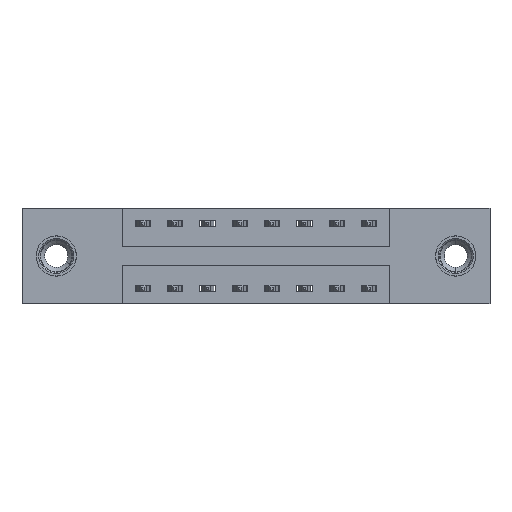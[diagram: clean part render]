
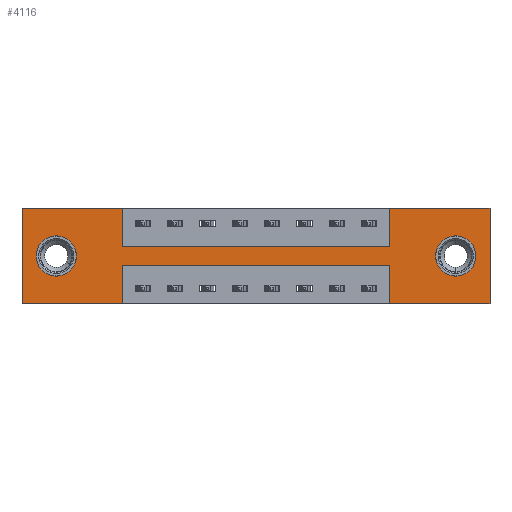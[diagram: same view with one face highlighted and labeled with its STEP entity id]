
A CAD part, front view. The second image highlights one B-rep face of the part: STEP entity #4116.
In plain terms, the highlighted planar face has unit normal (0, -1, 0).
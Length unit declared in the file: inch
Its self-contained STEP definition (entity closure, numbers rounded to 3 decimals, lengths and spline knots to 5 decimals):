
#4 = ORIENTED_EDGE ( 'NONE', *, *, #4979, .F. ) ;
#27 = CARTESIAN_POINT ( 'NONE',  ( 0., 0., -0.37 ) ) ;
#252 = LINE ( 'NONE', #2544, #3985 ) ;
#310 = LINE ( 'NONE', #9482, #10179 ) ;
#577 = ORIENTED_EDGE ( 'NONE', *, *, #8491, .F. ) ;
#803 = VECTOR ( 'NONE', #3928, 39.37008 ) ;
#817 = DIRECTION ( 'NONE',  ( 0., 0., 1. ) ) ;
#970 = AXIS2_PLACEMENT_3D ( 'NONE', #9080, #3993, #2358 ) ;
#1025 = CARTESIAN_POINT ( 'NONE',  ( 1.4225, 0., -0.37 ) ) ;
#1041 = ORIENTED_EDGE ( 'NONE', *, *, #8080, .F. ) ;
#1174 = CARTESIAN_POINT ( 'NONE',  ( 1.81, 0., 0. ) ) ;
#1250 = EDGE_CURVE ( 'NONE', #7081, #10296, #3600, .T. ) ;
#1262 = CARTESIAN_POINT ( 'NONE',  ( 0., 0., 0. ) ) ;
#1289 = ORIENTED_EDGE ( 'NONE', *, *, #5564, .F. ) ;
#1310 = CARTESIAN_POINT ( 'NONE',  ( 1.4225, 0., 0. ) ) ;
#1351 = CARTESIAN_POINT ( 'NONE',  ( 0.1325, 0., -0.185 ) ) ;
#1687 = CIRCLE ( 'NONE', #8643, 0.078 ) ;
#1735 = LINE ( 'NONE', #1174, #8257 ) ;
#1762 = ORIENTED_EDGE ( 'NONE', *, *, #9929, .F. ) ;
#1812 = DIRECTION ( 'NONE',  ( -1., 0., 0. ) ) ;
#1877 = VERTEX_POINT ( 'NONE', #9160 ) ;
#2152 = DIRECTION ( 'NONE',  ( 0., 1., 0. ) ) ;
#2358 = DIRECTION ( 'NONE',  ( 0., 0., 1. ) ) ;
#2379 = ORIENTED_EDGE ( 'NONE', *, *, #8146, .F. ) ;
#2544 = CARTESIAN_POINT ( 'NONE',  ( 0., 0., 0. ) ) ;
#2576 = CARTESIAN_POINT ( 'NONE',  ( 1.6775, 0., -0.185 ) ) ;
#2598 = EDGE_CURVE ( 'NONE', #11024, #10884, #2639, .T. ) ;
#2613 = CIRCLE ( 'NONE', #4164, 0.078 ) ;
#2615 = CARTESIAN_POINT ( 'NONE',  ( 1.4225, 0., 0. ) ) ;
#2639 = CIRCLE ( 'NONE', #5781, 0.078 ) ;
#2711 = VECTOR ( 'NONE', #8893, 39.37008 ) ;
#2727 = CARTESIAN_POINT ( 'NONE',  ( 0.1325, 0., -0.107 ) ) ;
#2881 = VECTOR ( 'NONE', #817, 39.37008 ) ;
#2910 = ORIENTED_EDGE ( 'NONE', *, *, #4052, .F. ) ;
#2995 = DIRECTION ( 'NONE',  ( 0., 0., 1. ) ) ;
#3021 = DIRECTION ( 'NONE',  ( 0., 1., 0. ) ) ;
#3043 = VERTEX_POINT ( 'NONE', #1025 ) ;
#3366 = DIRECTION ( 'NONE',  ( 0., -1., 0. ) ) ;
#3600 = LINE ( 'NONE', #3935, #6920 ) ;
#3783 = AXIS2_PLACEMENT_3D ( 'NONE', #27, #3366, #5979 ) ;
#3785 = EDGE_CURVE ( 'NONE', #10884, #11024, #2613, .T. ) ;
#3799 = DIRECTION ( 'NONE',  ( 1., 0., 0. ) ) ;
#3928 = DIRECTION ( 'NONE',  ( -1., 0., 0. ) ) ;
#3935 = CARTESIAN_POINT ( 'NONE',  ( 0.3875, 0., -0.37 ) ) ;
#3985 = VECTOR ( 'NONE', #8494, 39.37008 ) ;
#3993 = DIRECTION ( 'NONE',  ( 0., 1., 0. ) ) ;
#4052 = EDGE_CURVE ( 'NONE', #3043, #4626, #8217, .T. ) ;
#4082 = CARTESIAN_POINT ( 'NONE',  ( 0.3875, 0., -0.15 ) ) ;
#4116 = ADVANCED_FACE ( 'NONE', ( #9292, #9939, #6868 ), #10155, .T. ) ;
#4138 = CARTESIAN_POINT ( 'NONE',  ( 1.4225, 0., -0.37 ) ) ;
#4164 = AXIS2_PLACEMENT_3D ( 'NONE', #8963, #2152, #7339 ) ;
#4240 = VERTEX_POINT ( 'NONE', #6987 ) ;
#4421 = CARTESIAN_POINT ( 'NONE',  ( 0.3875, 0., -0.15 ) ) ;
#4422 = CARTESIAN_POINT ( 'NONE',  ( 0., 0., 0. ) ) ;
#4454 = LINE ( 'NONE', #1310, #5899 ) ;
#4476 = EDGE_CURVE ( 'NONE', #6394, #10966, #1687, .T. ) ;
#4532 = DIRECTION ( 'NONE',  ( 0., 0., -1. ) ) ;
#4626 = VERTEX_POINT ( 'NONE', #7547 ) ;
#4632 = CARTESIAN_POINT ( 'NONE',  ( 0.1325, 0., -0.263 ) ) ;
#4727 = ORIENTED_EDGE ( 'NONE', *, *, #3785, .T. ) ;
#4742 = VERTEX_POINT ( 'NONE', #8520 ) ;
#4807 = DIRECTION ( 'NONE',  ( 0., 0., -1. ) ) ;
#4900 = EDGE_CURVE ( 'NONE', #4742, #6120, #9551, .T. ) ;
#4979 = EDGE_CURVE ( 'NONE', #7237, #4742, #5648, .T. ) ;
#5195 = LINE ( 'NONE', #8920, #803 ) ;
#5290 = DIRECTION ( 'NONE',  ( 1., 0., 0. ) ) ;
#5388 = CARTESIAN_POINT ( 'NONE',  ( 0., 0., -0.37 ) ) ;
#5518 = ORIENTED_EDGE ( 'NONE', *, *, #2598, .T. ) ;
#5527 = VECTOR ( 'NONE', #4532, 39.37008 ) ;
#5564 = EDGE_CURVE ( 'NONE', #6120, #9863, #8842, .T. ) ;
#5648 = LINE ( 'NONE', #1262, #7539 ) ;
#5781 = AXIS2_PLACEMENT_3D ( 'NONE', #2576, #10335, #6895 ) ;
#5830 = CARTESIAN_POINT ( 'NONE',  ( 0.3875, 0., -0.37 ) ) ;
#5850 = CARTESIAN_POINT ( 'NONE',  ( 0.3875, 0., -0.22 ) ) ;
#5899 = VECTOR ( 'NONE', #10069, 39.37008 ) ;
#5979 = DIRECTION ( 'NONE',  ( 0., 0., -1. ) ) ;
#6120 = VERTEX_POINT ( 'NONE', #4421 ) ;
#6195 = CIRCLE ( 'NONE', #970, 0.078 ) ;
#6284 = EDGE_LOOP ( 'NONE', ( #5518, #4727 ) ) ;
#6394 = VERTEX_POINT ( 'NONE', #4632 ) ;
#6531 = ORIENTED_EDGE ( 'NONE', *, *, #4476, .T. ) ;
#6647 = ORIENTED_EDGE ( 'NONE', *, *, #10310, .F. ) ;
#6750 = EDGE_LOOP ( 'NONE', ( #6873, #2379, #2910, #577, #1041, #1762, #6647, #1289, #9093, #4, #9134, #6837 ) ) ;
#6837 = ORIENTED_EDGE ( 'NONE', *, *, #9474, .F. ) ;
#6861 = ORIENTED_EDGE ( 'NONE', *, *, #9233, .T. ) ;
#6868 = FACE_OUTER_BOUND ( 'NONE', #6750, .T. ) ;
#6873 = ORIENTED_EDGE ( 'NONE', *, *, #1250, .F. ) ;
#6895 = DIRECTION ( 'NONE',  ( 0., 0., -1. ) ) ;
#6920 = VECTOR ( 'NONE', #9895, 39.37008 ) ;
#6973 = CARTESIAN_POINT ( 'NONE',  ( 0.3875, 0., 0. ) ) ;
#6987 = CARTESIAN_POINT ( 'NONE',  ( 0., 0., -0.37 ) ) ;
#7081 = VERTEX_POINT ( 'NONE', #5850 ) ;
#7237 = VERTEX_POINT ( 'NONE', #4422 ) ;
#7339 = DIRECTION ( 'NONE',  ( 0., 0., -1. ) ) ;
#7539 = VECTOR ( 'NONE', #3799, 39.37008 ) ;
#7547 = CARTESIAN_POINT ( 'NONE',  ( 1.4225, 0., -0.22 ) ) ;
#7689 = CARTESIAN_POINT ( 'NONE',  ( 1.81, 0., -0.37 ) ) ;
#7787 = LINE ( 'NONE', #9625, #8823 ) ;
#8072 = EDGE_LOOP ( 'NONE', ( #6861, #6531 ) ) ;
#8080 = EDGE_CURVE ( 'NONE', #1877, #9260, #1735, .T. ) ;
#8146 = EDGE_CURVE ( 'NONE', #4626, #7081, #5195, .T. ) ;
#8217 = LINE ( 'NONE', #4138, #2881 ) ;
#8257 = VECTOR ( 'NONE', #4807, 39.37008 ) ;
#8386 = EDGE_CURVE ( 'NONE', #4240, #7237, #252, .T. ) ;
#8491 = EDGE_CURVE ( 'NONE', #9260, #3043, #7787, .T. ) ;
#8494 = DIRECTION ( 'NONE',  ( 0., 0., 1. ) ) ;
#8520 = CARTESIAN_POINT ( 'NONE',  ( 0.3875, 0., 0. ) ) ;
#8643 = AXIS2_PLACEMENT_3D ( 'NONE', #1351, #3021, #2995 ) ;
#8823 = VECTOR ( 'NONE', #1812, 39.37008 ) ;
#8842 = LINE ( 'NONE', #4082, #10834 ) ;
#8846 = LINE ( 'NONE', #5388, #2711 ) ;
#8893 = DIRECTION ( 'NONE',  ( -1., 0., 0. ) ) ;
#8920 = CARTESIAN_POINT ( 'NONE',  ( 0.3875, 0., -0.22 ) ) ;
#8963 = CARTESIAN_POINT ( 'NONE',  ( 1.6775, 0., -0.185 ) ) ;
#9080 = CARTESIAN_POINT ( 'NONE',  ( 0.1325, 0., -0.185 ) ) ;
#9093 = ORIENTED_EDGE ( 'NONE', *, *, #4900, .F. ) ;
#9134 = ORIENTED_EDGE ( 'NONE', *, *, #8386, .F. ) ;
#9160 = CARTESIAN_POINT ( 'NONE',  ( 1.81, 0., 0. ) ) ;
#9233 = EDGE_CURVE ( 'NONE', #10966, #6394, #6195, .T. ) ;
#9260 = VERTEX_POINT ( 'NONE', #7689 ) ;
#9292 = FACE_BOUND ( 'NONE', #6284, .T. ) ;
#9474 = EDGE_CURVE ( 'NONE', #10296, #4240, #8846, .T. ) ;
#9482 = CARTESIAN_POINT ( 'NONE',  ( 0., 0., 0. ) ) ;
#9551 = LINE ( 'NONE', #6973, #5527 ) ;
#9625 = CARTESIAN_POINT ( 'NONE',  ( 0., 0., -0.37 ) ) ;
#9863 = VERTEX_POINT ( 'NONE', #10032 ) ;
#9895 = DIRECTION ( 'NONE',  ( 0., 0., -1. ) ) ;
#9929 = EDGE_CURVE ( 'NONE', #10652, #1877, #310, .T. ) ;
#9939 = FACE_BOUND ( 'NONE', #8072, .T. ) ;
#10032 = CARTESIAN_POINT ( 'NONE',  ( 1.4225, 0., -0.15 ) ) ;
#10069 = DIRECTION ( 'NONE',  ( 0., 0., 1. ) ) ;
#10103 = CARTESIAN_POINT ( 'NONE',  ( 1.6775, 0., -0.263 ) ) ;
#10155 = PLANE ( 'NONE',  #3783 ) ;
#10179 = VECTOR ( 'NONE', #5290, 39.37008 ) ;
#10255 = CARTESIAN_POINT ( 'NONE',  ( 1.6775, 0., -0.107 ) ) ;
#10296 = VERTEX_POINT ( 'NONE', #5830 ) ;
#10310 = EDGE_CURVE ( 'NONE', #9863, #10652, #4454, .T. ) ;
#10335 = DIRECTION ( 'NONE',  ( 0., 1., 0. ) ) ;
#10652 = VERTEX_POINT ( 'NONE', #2615 ) ;
#10834 = VECTOR ( 'NONE', #10975, 39.37008 ) ;
#10884 = VERTEX_POINT ( 'NONE', #10103 ) ;
#10966 = VERTEX_POINT ( 'NONE', #2727 ) ;
#10975 = DIRECTION ( 'NONE',  ( 1., 0., 0. ) ) ;
#11024 = VERTEX_POINT ( 'NONE', #10255 ) ;
